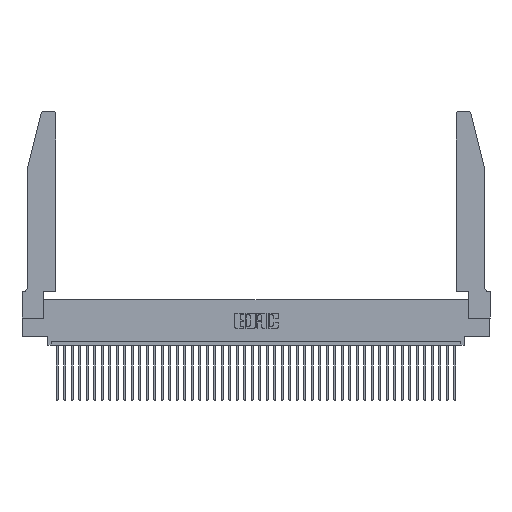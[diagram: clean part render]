
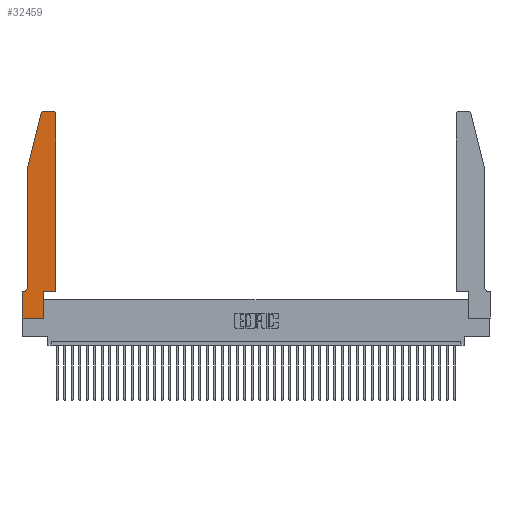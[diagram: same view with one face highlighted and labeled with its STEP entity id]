
A CAD part, top view. The second image highlights one B-rep face of the part: STEP entity #32459.
In plain terms, the highlighted planar face has unit normal (0, 0, 1).
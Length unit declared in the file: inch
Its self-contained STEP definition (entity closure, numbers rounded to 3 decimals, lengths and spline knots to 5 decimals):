
#18 = DIRECTION ( 'NONE',  ( 0., 0., 1. ) ) ;
#558 = DIRECTION ( 'NONE',  ( 1., 0., 0. ) ) ;
#873 = AXIS2_PLACEMENT_3D ( 'NONE', #9126, #22798, #25884 ) ;
#1707 = CARTESIAN_POINT ( 'NONE',  ( 0., 0., 0.37 ) ) ;
#1771 = VERTEX_POINT ( 'NONE', #20714 ) ;
#2861 = EDGE_CURVE ( 'NONE', #24071, #6763, #43276, .T. ) ;
#2917 = VECTOR ( 'NONE', #34213, 39.37008 ) ;
#3195 = ORIENTED_EDGE ( 'NONE', *, *, #19357, .T. ) ;
#3227 = CARTESIAN_POINT ( 'NONE',  ( 0.0755, 0.35, 0.37 ) ) ;
#3277 = DIRECTION ( 'NONE',  ( 0., 1., 0. ) ) ;
#4209 = LINE ( 'NONE', #3227, #41377 ) ;
#4472 = CARTESIAN_POINT ( 'NONE',  ( 0.2605, 2.75, 0.37 ) ) ;
#4672 = VERTEX_POINT ( 'NONE', #23597 ) ;
#4675 = LINE ( 'NONE', #23589, #40230 ) ;
#4855 = CARTESIAN_POINT ( 'NONE',  ( 0.0755, 2., 0.37 ) ) ;
#5070 = VERTEX_POINT ( 'NONE', #18283 ) ;
#5134 = CIRCLE ( 'NONE', #873, 0.07 ) ;
#5308 = VERTEX_POINT ( 'NONE', #18322 ) ;
#5534 = CIRCLE ( 'NONE', #12624, 0.03 ) ;
#5804 = AXIS2_PLACEMENT_3D ( 'NONE', #35136, #42469, #14837 ) ;
#5973 = EDGE_CURVE ( 'NONE', #19565, #22479, #4209, .T. ) ;
#6192 = CARTESIAN_POINT ( 'NONE',  ( 0.0055, 0.35, 0.37 ) ) ;
#6525 = EDGE_CURVE ( 'NONE', #26515, #5308, #12117, .T. ) ;
#6763 = VERTEX_POINT ( 'NONE', #16158 ) ;
#8012 = DIRECTION ( 'NONE',  ( -0.239, -0.971, 0. ) ) ;
#8634 = ORIENTED_EDGE ( 'NONE', *, *, #6525, .T. ) ;
#8931 = CARTESIAN_POINT ( 'NONE',  ( 0.4205, 2.75, 0.37 ) ) ;
#9126 = CARTESIAN_POINT ( 'NONE',  ( 0.0055, 0.42, 0.37 ) ) ;
#9282 = LINE ( 'NONE', #9515, #2917 ) ;
#9515 = CARTESIAN_POINT ( 'NONE',  ( 0., 0., 0.37 ) ) ;
#9992 = ORIENTED_EDGE ( 'NONE', *, *, #37391, .T. ) ;
#11115 = DIRECTION ( 'NONE',  ( 0., 1., 0. ) ) ;
#11592 = VECTOR ( 'NONE', #11115, 39.37008 ) ;
#12117 = LINE ( 'NONE', #17466, #11592 ) ;
#12624 = AXIS2_PLACEMENT_3D ( 'NONE', #42950, #17507, #558 ) ;
#12902 = CARTESIAN_POINT ( 'NONE',  ( 0.0755, 0.42, 0.37 ) ) ;
#14837 = DIRECTION ( 'NONE',  ( 1., 0., 0. ) ) ;
#16158 = CARTESIAN_POINT ( 'NONE',  ( 0.25487, 2.72718, 0.37 ) ) ;
#16232 = ORIENTED_EDGE ( 'NONE', *, *, #22570, .T. ) ;
#17013 = CARTESIAN_POINT ( 'NONE',  ( 0.284, 2.72, 0.37 ) ) ;
#17466 = CARTESIAN_POINT ( 'NONE',  ( 0.4505, 0.35, 0.37 ) ) ;
#17507 = DIRECTION ( 'NONE',  ( 0., 0., 1. ) ) ;
#18283 = CARTESIAN_POINT ( 'NONE',  ( 0.2865, 0., 0.37 ) ) ;
#18322 = CARTESIAN_POINT ( 'NONE',  ( 0.4505, 2.72, 0.37 ) ) ;
#19357 = EDGE_CURVE ( 'NONE', #21798, #19565, #5134, .T. ) ;
#19565 = VERTEX_POINT ( 'NONE', #6192 ) ;
#20316 = LINE ( 'NONE', #36734, #39369 ) ;
#20436 = LINE ( 'NONE', #4855, #42759 ) ;
#20714 = CARTESIAN_POINT ( 'NONE',  ( 0.0755, 2., 0.37 ) ) ;
#20997 = ORIENTED_EDGE ( 'NONE', *, *, #21510, .T. ) ;
#21510 = EDGE_CURVE ( 'NONE', #36946, #24071, #39006, .T. ) ;
#21789 = ORIENTED_EDGE ( 'NONE', *, *, #41626, .T. ) ;
#21798 = VERTEX_POINT ( 'NONE', #12902 ) ;
#21841 = PLANE ( 'NONE',  #5804 ) ;
#21853 = DIRECTION ( 'NONE',  ( -1., 0., 0. ) ) ;
#22223 = CARTESIAN_POINT ( 'NONE',  ( 0.4505, 0.35, 0.37 ) ) ;
#22304 = EDGE_CURVE ( 'NONE', #1771, #21798, #20436, .T. ) ;
#22479 = VERTEX_POINT ( 'NONE', #24143 ) ;
#22538 = CARTESIAN_POINT ( 'NONE',  ( 0.284, 2.75, 0.37 ) ) ;
#22570 = EDGE_CURVE ( 'NONE', #36180, #5070, #9282, .T. ) ;
#22798 = DIRECTION ( 'NONE',  ( 0., 0., -1. ) ) ;
#23170 = VECTOR ( 'NONE', #21853, 39.37008 ) ;
#23529 = EDGE_CURVE ( 'NONE', #5070, #4672, #20316, .T. ) ;
#23556 = CARTESIAN_POINT ( 'NONE',  ( 0.4505, 0.35, 0.37 ) ) ;
#23589 = CARTESIAN_POINT ( 'NONE',  ( 0., 0., 0.37 ) ) ;
#23597 = CARTESIAN_POINT ( 'NONE',  ( 0.2865, 0.35, 0.37 ) ) ;
#23715 = EDGE_CURVE ( 'NONE', #4672, #26515, #31361, .T. ) ;
#24071 = VERTEX_POINT ( 'NONE', #22538 ) ;
#24143 = CARTESIAN_POINT ( 'NONE',  ( 0., 0.35, 0.37 ) ) ;
#24189 = ORIENTED_EDGE ( 'NONE', *, *, #2861, .T. ) ;
#24480 = VECTOR ( 'NONE', #38448, 39.37008 ) ;
#25391 = CARTESIAN_POINT ( 'NONE',  ( 0.0755, 2., 0.37 ) ) ;
#25884 = DIRECTION ( 'NONE',  ( -1., 0., 0. ) ) ;
#26515 = VERTEX_POINT ( 'NONE', #23556 ) ;
#29408 = FACE_OUTER_BOUND ( 'NONE', #34499, .T. ) ;
#30677 = DIRECTION ( 'NONE',  ( 0., -1., 0. ) ) ;
#31361 = LINE ( 'NONE', #22223, #24480 ) ;
#31594 = EDGE_CURVE ( 'NONE', #5308, #36946, #5534, .T. ) ;
#32459 = ADVANCED_FACE ( 'NONE', ( #29408 ), #21841, .T. ) ;
#34095 = VECTOR ( 'NONE', #8012, 39.37008 ) ;
#34213 = DIRECTION ( 'NONE',  ( 1., 0., 0. ) ) ;
#34499 = EDGE_LOOP ( 'NONE', ( #20997, #24189, #9992, #37791, #3195, #37057, #21789, #16232, #36554, #43421, #8634, #43693 ) ) ;
#35136 = CARTESIAN_POINT ( 'NONE',  ( 0., 0.35, 0.37 ) ) ;
#35678 = DIRECTION ( 'NONE',  ( 0., -1., 0. ) ) ;
#36180 = VERTEX_POINT ( 'NONE', #1707 ) ;
#36554 = ORIENTED_EDGE ( 'NONE', *, *, #23529, .T. ) ;
#36734 = CARTESIAN_POINT ( 'NONE',  ( 0.2865, 0.35, 0.37 ) ) ;
#36946 = VERTEX_POINT ( 'NONE', #8931 ) ;
#37057 = ORIENTED_EDGE ( 'NONE', *, *, #5973, .T. ) ;
#37391 = EDGE_CURVE ( 'NONE', #6763, #1771, #38278, .T. ) ;
#37791 = ORIENTED_EDGE ( 'NONE', *, *, #22304, .T. ) ;
#38278 = LINE ( 'NONE', #25391, #34095 ) ;
#38448 = DIRECTION ( 'NONE',  ( 1., 0., 0. ) ) ;
#39006 = LINE ( 'NONE', #4472, #23170 ) ;
#39369 = VECTOR ( 'NONE', #3277, 39.37008 ) ;
#39824 = DIRECTION ( 'NONE',  ( -1., 0., 0. ) ) ;
#40230 = VECTOR ( 'NONE', #30677, 39.37008 ) ;
#40877 = DIRECTION ( 'NONE',  ( 1., 0., 0. ) ) ;
#41377 = VECTOR ( 'NONE', #39824, 39.37008 ) ;
#41626 = EDGE_CURVE ( 'NONE', #22479, #36180, #4675, .T. ) ;
#42469 = DIRECTION ( 'NONE',  ( 0., 0., 1. ) ) ;
#42759 = VECTOR ( 'NONE', #35678, 39.37008 ) ;
#42950 = CARTESIAN_POINT ( 'NONE',  ( 0.4205, 2.72, 0.37 ) ) ;
#43276 = CIRCLE ( 'NONE', #43530, 0.03 ) ;
#43421 = ORIENTED_EDGE ( 'NONE', *, *, #23715, .T. ) ;
#43530 = AXIS2_PLACEMENT_3D ( 'NONE', #17013, #18, #40877 ) ;
#43693 = ORIENTED_EDGE ( 'NONE', *, *, #31594, .T. ) ;
